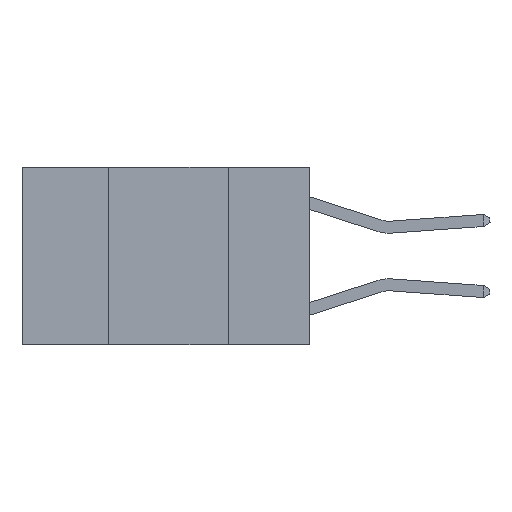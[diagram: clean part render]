
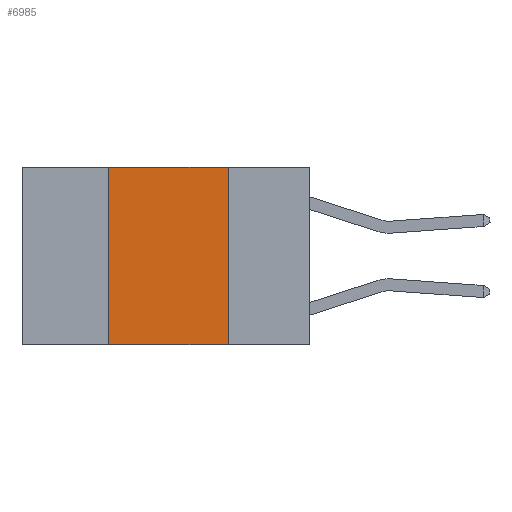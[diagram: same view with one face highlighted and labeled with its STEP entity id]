
A CAD part, left-side view. The second image highlights one B-rep face of the part: STEP entity #6985.
In plain terms, the highlighted planar face has unit normal (-1, 0, 0).
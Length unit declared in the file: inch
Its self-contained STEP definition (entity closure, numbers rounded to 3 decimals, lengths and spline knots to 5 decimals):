
#108 = ORIENTED_EDGE ( 'NONE', *, *, #8520, .T. ) ;
#115 = CARTESIAN_POINT ( 'NONE',  ( 0., 0.6, 0. ) ) ;
#302 = CARTESIAN_POINT ( 'NONE',  ( 0., 0.42, 0. ) ) ;
#447 = CARTESIAN_POINT ( 'NONE',  ( 0., 0.42, -0.37 ) ) ;
#490 = EDGE_LOOP ( 'NONE', ( #9289, #11601, #7217, #108 ) ) ;
#847 = DIRECTION ( 'NONE',  ( 0., 0., 1. ) ) ;
#1257 = VECTOR ( 'NONE', #2991, 39.37008 ) ;
#1558 = EDGE_CURVE ( 'NONE', #3867, #8875, #11629, .T. ) ;
#1813 = CARTESIAN_POINT ( 'NONE',  ( 0., 0.42, 0. ) ) ;
#2746 = LINE ( 'NONE', #9860, #11731 ) ;
#2832 = VERTEX_POINT ( 'NONE', #302 ) ;
#2871 = CARTESIAN_POINT ( 'NONE',  ( 0., 0.17, 0. ) ) ;
#2917 = DIRECTION ( 'NONE',  ( 1., 0., 0. ) ) ;
#2991 = DIRECTION ( 'NONE',  ( 0., -1., 0. ) ) ;
#3756 = FACE_OUTER_BOUND ( 'NONE', #490, .T. ) ;
#3867 = VERTEX_POINT ( 'NONE', #2871 ) ;
#3955 = EDGE_CURVE ( 'NONE', #2832, #3867, #8288, .T. ) ;
#6985 = ADVANCED_FACE ( 'NONE', ( #3756 ), #10996, .F. ) ;
#7217 = ORIENTED_EDGE ( 'NONE', *, *, #7952, .F. ) ;
#7242 = VECTOR ( 'NONE', #11259, 39.37008 ) ;
#7696 = VERTEX_POINT ( 'NONE', #447 ) ;
#7952 = EDGE_CURVE ( 'NONE', #7696, #2832, #11065, .T. ) ;
#8214 = VECTOR ( 'NONE', #847, 39.37008 ) ;
#8288 = LINE ( 'NONE', #8478, #1257 ) ;
#8478 = CARTESIAN_POINT ( 'NONE',  ( 0., 0.6, 0. ) ) ;
#8520 = EDGE_CURVE ( 'NONE', #7696, #8875, #2746, .T. ) ;
#8636 = CARTESIAN_POINT ( 'NONE',  ( 0., 0.17, 0. ) ) ;
#8875 = VERTEX_POINT ( 'NONE', #9165 ) ;
#9165 = CARTESIAN_POINT ( 'NONE',  ( 0., 0.17, -0.37 ) ) ;
#9289 = ORIENTED_EDGE ( 'NONE', *, *, #1558, .F. ) ;
#9297 = DIRECTION ( 'NONE',  ( 0., 0., -1. ) ) ;
#9860 = CARTESIAN_POINT ( 'NONE',  ( 0., 0.6, -0.37 ) ) ;
#10681 = DIRECTION ( 'NONE',  ( 0., -1., 0. ) ) ;
#10996 = PLANE ( 'NONE',  #11229 ) ;
#11065 = LINE ( 'NONE', #1813, #8214 ) ;
#11229 = AXIS2_PLACEMENT_3D ( 'NONE', #115, #2917, #9297 ) ;
#11259 = DIRECTION ( 'NONE',  ( 0., 0., -1. ) ) ;
#11601 = ORIENTED_EDGE ( 'NONE', *, *, #3955, .F. ) ;
#11629 = LINE ( 'NONE', #8636, #7242 ) ;
#11731 = VECTOR ( 'NONE', #10681, 39.37008 ) ;
